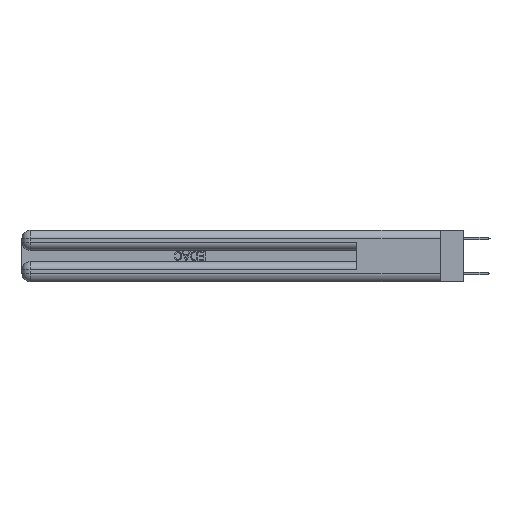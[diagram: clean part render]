
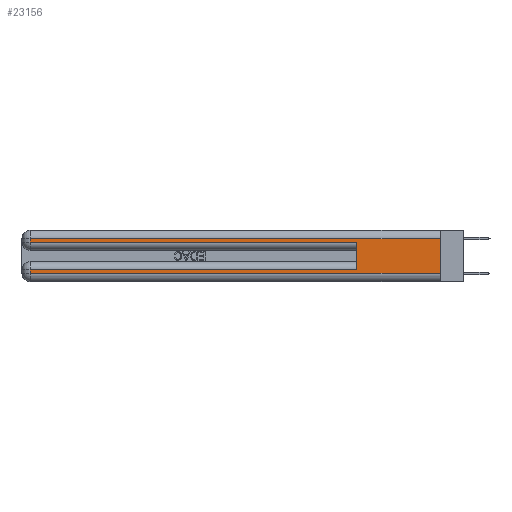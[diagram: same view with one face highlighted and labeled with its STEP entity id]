
A CAD part, left-side view. The second image highlights one B-rep face of the part: STEP entity #23156.
In plain terms, the highlighted planar face has unit normal (-1, 0, 0).
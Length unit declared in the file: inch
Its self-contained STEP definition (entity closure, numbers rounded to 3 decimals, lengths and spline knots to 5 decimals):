
#69 = LINE ( 'NONE', #23408, #12154 ) ;
#891 = VERTEX_POINT ( 'NONE', #24354 ) ;
#1166 = DIRECTION ( 'NONE',  ( 0., 1., 0. ) ) ;
#1255 = DIRECTION ( 'NONE',  ( 0., 0., -1. ) ) ;
#1761 = CARTESIAN_POINT ( 'NONE',  ( 0., 2.94, 0.31 ) ) ;
#2853 = CARTESIAN_POINT ( 'NONE',  ( 0., 2.94, 0.285 ) ) ;
#4221 = VECTOR ( 'NONE', #1255, 39.37008 ) ;
#4836 = VERTEX_POINT ( 'NONE', #7764 ) ;
#5090 = ORIENTED_EDGE ( 'NONE', *, *, #8662, .T. ) ;
#5154 = DIRECTION ( 'NONE',  ( 0., 0., -1. ) ) ;
#5483 = ORIENTED_EDGE ( 'NONE', *, *, #10348, .T. ) ;
#5845 = CARTESIAN_POINT ( 'NONE',  ( 0., 0.6, 0.145 ) ) ;
#5930 = ORIENTED_EDGE ( 'NONE', *, *, #24726, .T. ) ;
#5960 = CARTESIAN_POINT ( 'NONE',  ( 0., 2.94, 0.085 ) ) ;
#6150 = VERTEX_POINT ( 'NONE', #2853 ) ;
#7764 = CARTESIAN_POINT ( 'NONE',  ( 0., 0., 0.31 ) ) ;
#8498 = ORIENTED_EDGE ( 'NONE', *, *, #11387, .T. ) ;
#8662 = EDGE_CURVE ( 'NONE', #25333, #891, #69, .T. ) ;
#8708 = LINE ( 'NONE', #13604, #19892 ) ;
#9095 = LINE ( 'NONE', #5845, #20272 ) ;
#9269 = DIRECTION ( 'NONE',  ( 0., 0., -1. ) ) ;
#9944 = DIRECTION ( 'NONE',  ( 0., -1., 0. ) ) ;
#9966 = EDGE_CURVE ( 'NONE', #4836, #891, #16912, .T. ) ;
#10348 = EDGE_CURVE ( 'NONE', #15295, #25333, #19352, .T. ) ;
#11061 = VERTEX_POINT ( 'NONE', #28186 ) ;
#11387 = EDGE_CURVE ( 'NONE', #6150, #18092, #16500, .T. ) ;
#12154 = VECTOR ( 'NONE', #9944, 39.37008 ) ;
#12522 = CARTESIAN_POINT ( 'NONE',  ( 0., 0., 0.37 ) ) ;
#13312 = CARTESIAN_POINT ( 'NONE',  ( 0., 0., 0.085 ) ) ;
#13604 = CARTESIAN_POINT ( 'NONE',  ( 0., 2.94, 0.37 ) ) ;
#15209 = FACE_OUTER_BOUND ( 'NONE', #23245, .T. ) ;
#15295 = VERTEX_POINT ( 'NONE', #5960 ) ;
#15705 = CARTESIAN_POINT ( 'NONE',  ( 0., 0., 0.285 ) ) ;
#15859 = DIRECTION ( 'NONE',  ( 0., 0., -1. ) ) ;
#16347 = PLANE ( 'NONE',  #20833 ) ;
#16500 = LINE ( 'NONE', #15705, #27785 ) ;
#16636 = ORIENTED_EDGE ( 'NONE', *, *, #24365, .T. ) ;
#16912 = LINE ( 'NONE', #12522, #4221 ) ;
#17464 = LINE ( 'NONE', #28197, #28733 ) ;
#18016 = DIRECTION ( 'NONE',  ( 0., -1., 0. ) ) ;
#18092 = VERTEX_POINT ( 'NONE', #19199 ) ;
#18593 = DIRECTION ( 'NONE',  ( 1., 0., 0. ) ) ;
#19199 = CARTESIAN_POINT ( 'NONE',  ( 0., 0.6, 0.285 ) ) ;
#19352 = LINE ( 'NONE', #27295, #24698 ) ;
#19680 = EDGE_CURVE ( 'NONE', #11061, #15295, #22801, .T. ) ;
#19892 = VECTOR ( 'NONE', #15859, 39.37008 ) ;
#20031 = EDGE_CURVE ( 'NONE', #11061, #18092, #9095, .T. ) ;
#20035 = ORIENTED_EDGE ( 'NONE', *, *, #9966, .F. ) ;
#20272 = VECTOR ( 'NONE', #23832, 39.37008 ) ;
#20833 = AXIS2_PLACEMENT_3D ( 'NONE', #25347, #18593, #5154 ) ;
#21971 = ORIENTED_EDGE ( 'NONE', *, *, #20031, .F. ) ;
#22772 = CARTESIAN_POINT ( 'NONE',  ( 0., 2.94, 0.06 ) ) ;
#22801 = LINE ( 'NONE', #13312, #28815 ) ;
#23156 = ADVANCED_FACE ( 'NONE', ( #15209 ), #16347, .F. ) ;
#23245 = EDGE_LOOP ( 'NONE', ( #20035, #5930, #16636, #8498, #21971, #28612, #5483, #5090 ) ) ;
#23408 = CARTESIAN_POINT ( 'NONE',  ( 0., 0., 0.06 ) ) ;
#23832 = DIRECTION ( 'NONE',  ( 0., 0., 1. ) ) ;
#24354 = CARTESIAN_POINT ( 'NONE',  ( 0., 0., 0.06 ) ) ;
#24365 = EDGE_CURVE ( 'NONE', #24921, #6150, #8708, .T. ) ;
#24698 = VECTOR ( 'NONE', #9269, 39.37008 ) ;
#24726 = EDGE_CURVE ( 'NONE', #4836, #24921, #17464, .T. ) ;
#24921 = VERTEX_POINT ( 'NONE', #1761 ) ;
#25333 = VERTEX_POINT ( 'NONE', #22772 ) ;
#25347 = CARTESIAN_POINT ( 'NONE',  ( 0., 0., 0.37 ) ) ;
#27295 = CARTESIAN_POINT ( 'NONE',  ( 0., 2.94, 0.37 ) ) ;
#27785 = VECTOR ( 'NONE', #18016, 39.37008 ) ;
#28186 = CARTESIAN_POINT ( 'NONE',  ( 0., 0.6, 0.085 ) ) ;
#28197 = CARTESIAN_POINT ( 'NONE',  ( 0., 0., 0.31 ) ) ;
#28612 = ORIENTED_EDGE ( 'NONE', *, *, #19680, .T. ) ;
#28733 = VECTOR ( 'NONE', #1166, 39.37008 ) ;
#28815 = VECTOR ( 'NONE', #29080, 39.37008 ) ;
#29080 = DIRECTION ( 'NONE',  ( 0., 1., 0. ) ) ;
